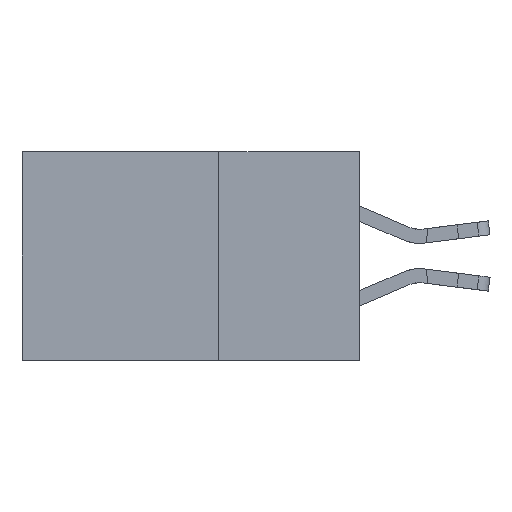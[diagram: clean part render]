
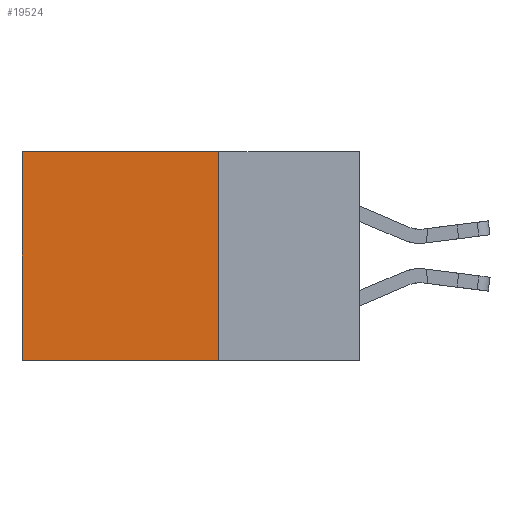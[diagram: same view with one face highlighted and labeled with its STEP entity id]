
A CAD part, left-side view. The second image highlights one B-rep face of the part: STEP entity #19524.
In plain terms, the highlighted planar face has unit normal (-1, 0, 0).
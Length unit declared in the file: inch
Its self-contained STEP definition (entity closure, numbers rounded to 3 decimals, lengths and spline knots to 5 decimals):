
#355 = VERTEX_POINT ( 'NONE', #15986 ) ;
#2102 = DIRECTION ( 'NONE',  ( 0., 1., 0. ) ) ;
#2655 = DIRECTION ( 'NONE',  ( 0., 1., 0. ) ) ;
#3799 = EDGE_CURVE ( 'NONE', #355, #17064, #20040, .T. ) ;
#4264 = DIRECTION ( 'NONE',  ( 1., 0., 0. ) ) ;
#5428 = EDGE_LOOP ( 'NONE', ( #16989, #7390, #6533, #8863 ) ) ;
#5595 = VECTOR ( 'NONE', #10626, 39.37008 ) ;
#5847 = CARTESIAN_POINT ( 'NONE',  ( 0.2875, 0.25, -0.37 ) ) ;
#6533 = ORIENTED_EDGE ( 'NONE', *, *, #18412, .F. ) ;
#6810 = CARTESIAN_POINT ( 'NONE',  ( 0.2875, 0.6, -0.37 ) ) ;
#7347 = PLANE ( 'NONE',  #9968 ) ;
#7384 = DIRECTION ( 'NONE',  ( 0., 0., -1. ) ) ;
#7390 = ORIENTED_EDGE ( 'NONE', *, *, #14904, .F. ) ;
#7622 = VERTEX_POINT ( 'NONE', #9373 ) ;
#7838 = EDGE_CURVE ( 'NONE', #10272, #355, #12243, .T. ) ;
#8631 = LINE ( 'NONE', #5847, #19959 ) ;
#8863 = ORIENTED_EDGE ( 'NONE', *, *, #7838, .T. ) ;
#8930 = CARTESIAN_POINT ( 'NONE',  ( 0.2875, 0.6, 0. ) ) ;
#9064 = CARTESIAN_POINT ( 'NONE',  ( 0.2875, 0.25, 0. ) ) ;
#9373 = CARTESIAN_POINT ( 'NONE',  ( 0.2875, 0.25, -0.37 ) ) ;
#9968 = AXIS2_PLACEMENT_3D ( 'NONE', #13581, #4264, #15119 ) ;
#10272 = VERTEX_POINT ( 'NONE', #11233 ) ;
#10626 = DIRECTION ( 'NONE',  ( 0., 0., -1. ) ) ;
#11233 = CARTESIAN_POINT ( 'NONE',  ( 0.2875, 0.25, 0. ) ) ;
#12243 = LINE ( 'NONE', #13047, #15856 ) ;
#13047 = CARTESIAN_POINT ( 'NONE',  ( 0.2875, 0.25, 0. ) ) ;
#13581 = CARTESIAN_POINT ( 'NONE',  ( 0.2875, 0.25, 0. ) ) ;
#13851 = LINE ( 'NONE', #9064, #5595 ) ;
#14904 = EDGE_CURVE ( 'NONE', #7622, #17064, #8631, .T. ) ;
#15119 = DIRECTION ( 'NONE',  ( 0., 0., -1. ) ) ;
#15424 = FACE_OUTER_BOUND ( 'NONE', #5428, .T. ) ;
#15856 = VECTOR ( 'NONE', #2102, 39.37008 ) ;
#15975 = VECTOR ( 'NONE', #7384, 39.37008 ) ;
#15986 = CARTESIAN_POINT ( 'NONE',  ( 0.2875, 0.6, 0. ) ) ;
#16989 = ORIENTED_EDGE ( 'NONE', *, *, #3799, .T. ) ;
#17064 = VERTEX_POINT ( 'NONE', #6810 ) ;
#18412 = EDGE_CURVE ( 'NONE', #10272, #7622, #13851, .T. ) ;
#19524 = ADVANCED_FACE ( 'NONE', ( #15424 ), #7347, .F. ) ;
#19959 = VECTOR ( 'NONE', #2655, 39.37008 ) ;
#20040 = LINE ( 'NONE', #8930, #15975 ) ;
